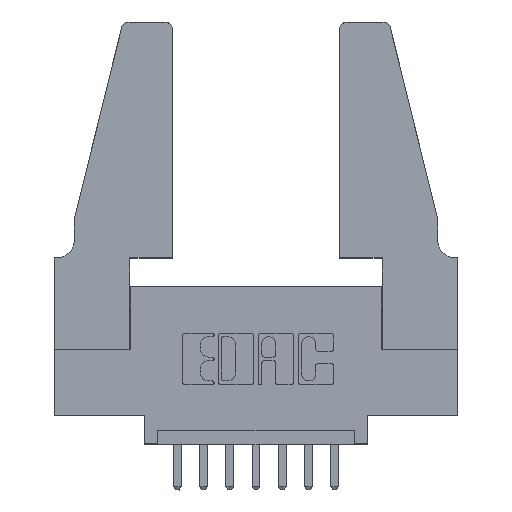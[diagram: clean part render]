
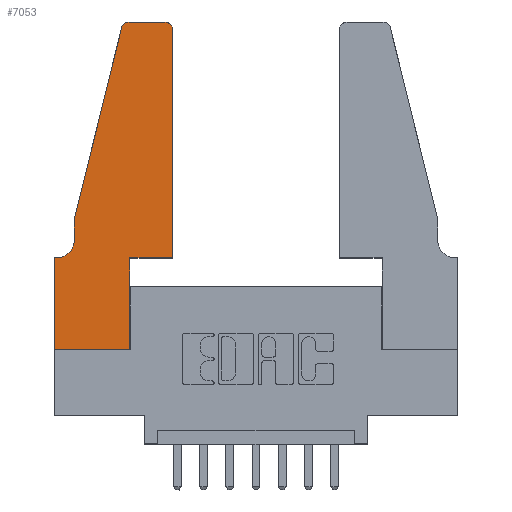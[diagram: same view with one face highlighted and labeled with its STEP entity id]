
A CAD part, top view. The second image highlights one B-rep face of the part: STEP entity #7053.
In plain terms, the highlighted planar face has unit normal (0, 0, 1).
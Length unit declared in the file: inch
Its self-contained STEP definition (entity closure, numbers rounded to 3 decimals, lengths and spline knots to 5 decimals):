
#299 = CARTESIAN_POINT ( 'NONE',  ( 0.0755, 0.5, 0.37 ) ) ;
#378 = AXIS2_PLACEMENT_3D ( 'NONE', #11899, #8373, #2656 ) ;
#384 = DIRECTION ( 'NONE',  ( 1., 0., 0. ) ) ;
#587 = LINE ( 'NONE', #299, #5380 ) ;
#778 = CARTESIAN_POINT ( 'NONE',  ( 0.0055, 0.42, 0.37 ) ) ;
#825 = CARTESIAN_POINT ( 'NONE',  ( 0., 0., 0.37 ) ) ;
#969 = DIRECTION ( 'NONE',  ( -0.239, -0.971, 0. ) ) ;
#1029 = EDGE_CURVE ( 'NONE', #11455, #10504, #8563, .T. ) ;
#1153 = CIRCLE ( 'NONE', #378, 0.03 ) ;
#1183 = DIRECTION ( 'NONE',  ( 0., -1., 0. ) ) ;
#1636 = CARTESIAN_POINT ( 'NONE',  ( 0.25487, 1.22718, 0.37 ) ) ;
#1770 = VECTOR ( 'NONE', #2035, 39.37008 ) ;
#2012 = ORIENTED_EDGE ( 'NONE', *, *, #7632, .T. ) ;
#2035 = DIRECTION ( 'NONE',  ( 0., -1., 0. ) ) ;
#2331 = EDGE_CURVE ( 'NONE', #8726, #3005, #9419, .T. ) ;
#2412 = LINE ( 'NONE', #11731, #6294 ) ;
#2541 = VERTEX_POINT ( 'NONE', #8179 ) ;
#2596 = EDGE_LOOP ( 'NONE', ( #9167, #10052, #6668, #8976, #2012, #12119, #12143, #11889, #9084, #8885, #4584, #9617 ) ) ;
#2614 = VERTEX_POINT ( 'NONE', #9669 ) ;
#2656 = DIRECTION ( 'NONE',  ( 1., 0., 0. ) ) ;
#2751 = LINE ( 'NONE', #3237, #7520 ) ;
#2826 = CARTESIAN_POINT ( 'NONE',  ( 0.0755, 0.5, 0.37 ) ) ;
#3005 = VERTEX_POINT ( 'NONE', #6735 ) ;
#3228 = DIRECTION ( 'NONE',  ( 1., 0., 0. ) ) ;
#3237 = CARTESIAN_POINT ( 'NONE',  ( 0.4505, 0.35, 0.37 ) ) ;
#3308 = CARTESIAN_POINT ( 'NONE',  ( 0., 0.35, 0.37 ) ) ;
#3488 = EDGE_CURVE ( 'NONE', #6928, #7006, #4913, .T. ) ;
#3568 = DIRECTION ( 'NONE',  ( 1., 0., 0. ) ) ;
#3669 = LINE ( 'NONE', #7152, #7826 ) ;
#4126 = CIRCLE ( 'NONE', #4501, 0.03 ) ;
#4156 = PLANE ( 'NONE',  #9489 ) ;
#4185 = FACE_OUTER_BOUND ( 'NONE', #2596, .T. ) ;
#4252 = VERTEX_POINT ( 'NONE', #11179 ) ;
#4317 = CARTESIAN_POINT ( 'NONE',  ( 0.0755, 0.42, 0.37 ) ) ;
#4408 = DIRECTION ( 'NONE',  ( 0., 0., 1. ) ) ;
#4501 = AXIS2_PLACEMENT_3D ( 'NONE', #10196, #4408, #3568 ) ;
#4584 = ORIENTED_EDGE ( 'NONE', *, *, #5830, .T. ) ;
#4714 = DIRECTION ( 'NONE',  ( 0., 0., -1. ) ) ;
#4782 = CARTESIAN_POINT ( 'NONE',  ( 0.0755, 0.5, 0.37 ) ) ;
#4791 = VECTOR ( 'NONE', #10005, 39.37008 ) ;
#4913 = LINE ( 'NONE', #825, #1770 ) ;
#5227 = CARTESIAN_POINT ( 'NONE',  ( 0., 0., 0.37 ) ) ;
#5347 = DIRECTION ( 'NONE',  ( -1., 0., 0. ) ) ;
#5380 = VECTOR ( 'NONE', #1183, 39.37008 ) ;
#5830 = EDGE_CURVE ( 'NONE', #8747, #4252, #2412, .T. ) ;
#6053 = VERTEX_POINT ( 'NONE', #12386 ) ;
#6294 = VECTOR ( 'NONE', #11638, 39.37008 ) ;
#6319 = EDGE_CURVE ( 'NONE', #10504, #9127, #587, .T. ) ;
#6345 = VECTOR ( 'NONE', #10808, 39.37008 ) ;
#6668 = ORIENTED_EDGE ( 'NONE', *, *, #1029, .T. ) ;
#6735 = CARTESIAN_POINT ( 'NONE',  ( 0.284, 1.25, 0.37 ) ) ;
#6835 = LINE ( 'NONE', #11896, #11603 ) ;
#6928 = VERTEX_POINT ( 'NONE', #10650 ) ;
#7006 = VERTEX_POINT ( 'NONE', #5227 ) ;
#7042 = DIRECTION ( 'NONE',  ( 0., 1., 0. ) ) ;
#7053 = ADVANCED_FACE ( 'NONE', ( #4185 ), #4156, .T. ) ;
#7152 = CARTESIAN_POINT ( 'NONE',  ( 0.0755, 0.35, 0.37 ) ) ;
#7514 = CARTESIAN_POINT ( 'NONE',  ( 0.4505, 0.35, 0.37 ) ) ;
#7520 = VECTOR ( 'NONE', #384, 39.37008 ) ;
#7632 = EDGE_CURVE ( 'NONE', #9127, #6053, #8183, .T. ) ;
#7642 = VECTOR ( 'NONE', #969, 39.37008 ) ;
#7726 = AXIS2_PLACEMENT_3D ( 'NONE', #778, #4714, #8391 ) ;
#7826 = VECTOR ( 'NONE', #5347, 39.37008 ) ;
#7885 = EDGE_CURVE ( 'NONE', #3005, #11455, #1153, .T. ) ;
#8116 = EDGE_CURVE ( 'NONE', #2541, #2614, #6835, .T. ) ;
#8179 = CARTESIAN_POINT ( 'NONE',  ( 0.2865, 0., 0.37 ) ) ;
#8183 = CIRCLE ( 'NONE', #7726, 0.07 ) ;
#8373 = DIRECTION ( 'NONE',  ( 0., 0., 1. ) ) ;
#8391 = DIRECTION ( 'NONE',  ( -1., 0., 0. ) ) ;
#8563 = LINE ( 'NONE', #4782, #7642 ) ;
#8726 = VERTEX_POINT ( 'NONE', #11452 ) ;
#8747 = VERTEX_POINT ( 'NONE', #7514 ) ;
#8885 = ORIENTED_EDGE ( 'NONE', *, *, #11572, .T. ) ;
#8944 = DIRECTION ( 'NONE',  ( 0., 0., 1. ) ) ;
#8976 = ORIENTED_EDGE ( 'NONE', *, *, #6319, .T. ) ;
#9004 = CARTESIAN_POINT ( 'NONE',  ( 0.2605, 1.25, 0.37 ) ) ;
#9084 = ORIENTED_EDGE ( 'NONE', *, *, #8116, .T. ) ;
#9127 = VERTEX_POINT ( 'NONE', #4317 ) ;
#9167 = ORIENTED_EDGE ( 'NONE', *, *, #2331, .T. ) ;
#9419 = LINE ( 'NONE', #9004, #4791 ) ;
#9489 = AXIS2_PLACEMENT_3D ( 'NONE', #3308, #8944, #3228 ) ;
#9617 = ORIENTED_EDGE ( 'NONE', *, *, #10854, .T. ) ;
#9669 = CARTESIAN_POINT ( 'NONE',  ( 0.2865, 0.35, 0.37 ) ) ;
#9772 = LINE ( 'NONE', #9845, #6345 ) ;
#9845 = CARTESIAN_POINT ( 'NONE',  ( 0., 0., 0.37 ) ) ;
#10005 = DIRECTION ( 'NONE',  ( -1., 0., 0. ) ) ;
#10052 = ORIENTED_EDGE ( 'NONE', *, *, #7885, .T. ) ;
#10196 = CARTESIAN_POINT ( 'NONE',  ( 0.4205, 1.22, 0.37 ) ) ;
#10504 = VERTEX_POINT ( 'NONE', #2826 ) ;
#10650 = CARTESIAN_POINT ( 'NONE',  ( 0., 0.35, 0.37 ) ) ;
#10808 = DIRECTION ( 'NONE',  ( 1., 0., 0. ) ) ;
#10854 = EDGE_CURVE ( 'NONE', #4252, #8726, #4126, .T. ) ;
#11167 = EDGE_CURVE ( 'NONE', #7006, #2541, #9772, .T. ) ;
#11179 = CARTESIAN_POINT ( 'NONE',  ( 0.4505, 1.22, 0.37 ) ) ;
#11274 = EDGE_CURVE ( 'NONE', #6053, #6928, #3669, .T. ) ;
#11452 = CARTESIAN_POINT ( 'NONE',  ( 0.4205, 1.25, 0.37 ) ) ;
#11455 = VERTEX_POINT ( 'NONE', #1636 ) ;
#11572 = EDGE_CURVE ( 'NONE', #2614, #8747, #2751, .T. ) ;
#11603 = VECTOR ( 'NONE', #7042, 39.37008 ) ;
#11638 = DIRECTION ( 'NONE',  ( 0., 1., 0. ) ) ;
#11731 = CARTESIAN_POINT ( 'NONE',  ( 0.4505, 0.35, 0.37 ) ) ;
#11889 = ORIENTED_EDGE ( 'NONE', *, *, #11167, .T. ) ;
#11896 = CARTESIAN_POINT ( 'NONE',  ( 0.2865, 0.35, 0.37 ) ) ;
#11899 = CARTESIAN_POINT ( 'NONE',  ( 0.284, 1.22, 0.37 ) ) ;
#12119 = ORIENTED_EDGE ( 'NONE', *, *, #11274, .T. ) ;
#12143 = ORIENTED_EDGE ( 'NONE', *, *, #3488, .T. ) ;
#12386 = CARTESIAN_POINT ( 'NONE',  ( 0.0055, 0.35, 0.37 ) ) ;
